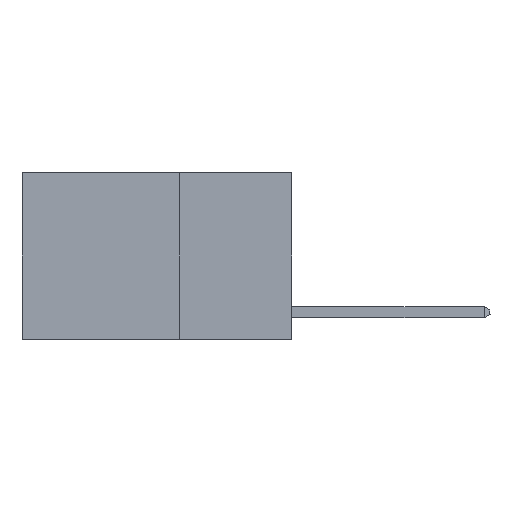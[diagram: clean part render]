
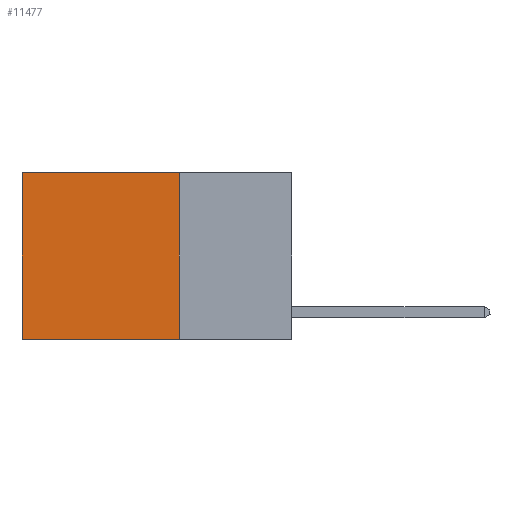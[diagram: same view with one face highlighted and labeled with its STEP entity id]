
A CAD part, left-side view. The second image highlights one B-rep face of the part: STEP entity #11477.
In plain terms, the highlighted planar face has unit normal (-1, 0, 0).
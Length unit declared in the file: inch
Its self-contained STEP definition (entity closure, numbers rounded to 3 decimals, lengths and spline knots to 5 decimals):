
#339 = VERTEX_POINT ( 'NONE', #15911 ) ;
#762 = ORIENTED_EDGE ( 'NONE', *, *, #6316, .F. ) ;
#1279 = DIRECTION ( 'NONE',  ( 0., 0., -1. ) ) ;
#1490 = EDGE_CURVE ( 'NONE', #6209, #339, #19370, .T. ) ;
#1567 = PLANE ( 'NONE',  #10114 ) ;
#3051 = EDGE_LOOP ( 'NONE', ( #13662, #22365, #762, #7830 ) ) ;
#3290 = CARTESIAN_POINT ( 'NONE',  ( 0.2625, 0.25, -0.37 ) ) ;
#5031 = VERTEX_POINT ( 'NONE', #11843 ) ;
#6209 = VERTEX_POINT ( 'NONE', #21447 ) ;
#6316 = EDGE_CURVE ( 'NONE', #6209, #10486, #7480, .T. ) ;
#7480 = LINE ( 'NONE', #23783, #22882 ) ;
#7830 = ORIENTED_EDGE ( 'NONE', *, *, #1490, .T. ) ;
#8408 = LINE ( 'NONE', #3290, #12523 ) ;
#9737 = DIRECTION ( 'NONE',  ( 1., 0., 0. ) ) ;
#10114 = AXIS2_PLACEMENT_3D ( 'NONE', #19764, #9737, #23745 ) ;
#10486 = VERTEX_POINT ( 'NONE', #24126 ) ;
#11477 = ADVANCED_FACE ( 'NONE', ( #11835 ), #1567, .F. ) ;
#11835 = FACE_OUTER_BOUND ( 'NONE', #3051, .T. ) ;
#11843 = CARTESIAN_POINT ( 'NONE',  ( 0.2625, 0.6, -0.37 ) ) ;
#12065 = EDGE_CURVE ( 'NONE', #339, #5031, #24947, .T. ) ;
#12523 = VECTOR ( 'NONE', #17427, 39.37008 ) ;
#12596 = CARTESIAN_POINT ( 'NONE',  ( 0.2625, 0.25, 0. ) ) ;
#13662 = ORIENTED_EDGE ( 'NONE', *, *, #12065, .T. ) ;
#13696 = VECTOR ( 'NONE', #1279, 39.37008 ) ;
#15474 = EDGE_CURVE ( 'NONE', #10486, #5031, #8408, .T. ) ;
#15911 = CARTESIAN_POINT ( 'NONE',  ( 0.2625, 0.6, 0. ) ) ;
#17427 = DIRECTION ( 'NONE',  ( 0., 1., 0. ) ) ;
#19370 = LINE ( 'NONE', #12596, #22800 ) ;
#19764 = CARTESIAN_POINT ( 'NONE',  ( 0.2625, 0.25, 0. ) ) ;
#21447 = CARTESIAN_POINT ( 'NONE',  ( 0.2625, 0.25, 0. ) ) ;
#21785 = DIRECTION ( 'NONE',  ( 0., 0., -1. ) ) ;
#22365 = ORIENTED_EDGE ( 'NONE', *, *, #15474, .F. ) ;
#22800 = VECTOR ( 'NONE', #24618, 39.37008 ) ;
#22882 = VECTOR ( 'NONE', #21785, 39.37008 ) ;
#23383 = CARTESIAN_POINT ( 'NONE',  ( 0.2625, 0.6, 0. ) ) ;
#23745 = DIRECTION ( 'NONE',  ( 0., 0., -1. ) ) ;
#23783 = CARTESIAN_POINT ( 'NONE',  ( 0.2625, 0.25, 0. ) ) ;
#24126 = CARTESIAN_POINT ( 'NONE',  ( 0.2625, 0.25, -0.37 ) ) ;
#24618 = DIRECTION ( 'NONE',  ( 0., 1., 0. ) ) ;
#24947 = LINE ( 'NONE', #23383, #13696 ) ;
